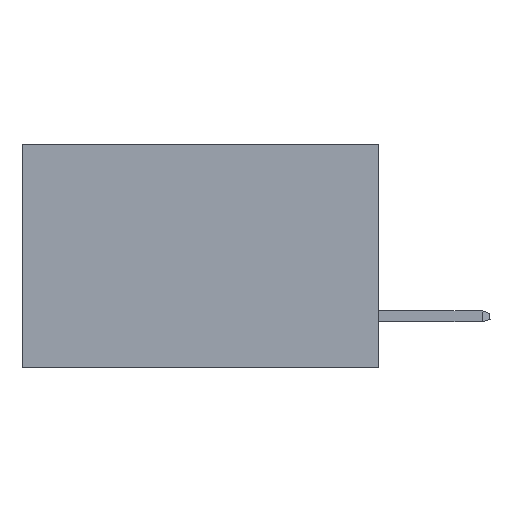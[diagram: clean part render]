
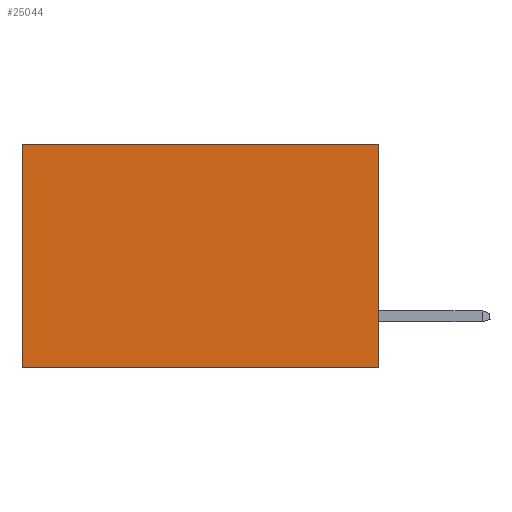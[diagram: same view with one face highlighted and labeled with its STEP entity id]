
A CAD part, left-side view. The second image highlights one B-rep face of the part: STEP entity #25044.
In plain terms, the highlighted planar face has unit normal (-1, 0, 0).
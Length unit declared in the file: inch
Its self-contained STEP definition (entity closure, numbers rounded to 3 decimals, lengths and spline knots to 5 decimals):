
#1061 = ORIENTED_EDGE ( 'NONE', *, *, #13146, .F. ) ;
#1868 = LINE ( 'NONE', #22021, #13992 ) ;
#2706 = CARTESIAN_POINT ( 'NONE',  ( 0.277, 0., 0. ) ) ;
#2955 = DIRECTION ( 'NONE',  ( 1., 0., 0. ) ) ;
#3081 = VERTEX_POINT ( 'NONE', #17607 ) ;
#4212 = VECTOR ( 'NONE', #24711, 39.37008 ) ;
#4604 = LINE ( 'NONE', #2706, #22909 ) ;
#5307 = EDGE_CURVE ( 'NONE', #3081, #27605, #1868, .T. ) ;
#7380 = CARTESIAN_POINT ( 'NONE',  ( 0.277, 0., 0. ) ) ;
#9707 = ORIENTED_EDGE ( 'NONE', *, *, #5307, .T. ) ;
#9942 = EDGE_CURVE ( 'NONE', #21710, #3081, #4604, .T. ) ;
#10630 = VECTOR ( 'NONE', #27394, 39.37008 ) ;
#10863 = FACE_OUTER_BOUND ( 'NONE', #11368, .T. ) ;
#10895 = CARTESIAN_POINT ( 'NONE',  ( 0.277, 0., -0.37 ) ) ;
#11368 = EDGE_LOOP ( 'NONE', ( #9707, #1061, #27638, #25913 ) ) ;
#13146 = EDGE_CURVE ( 'NONE', #21441, #27605, #15527, .T. ) ;
#13992 = VECTOR ( 'NONE', #22267, 39.37008 ) ;
#15527 = LINE ( 'NONE', #10895, #10630 ) ;
#17388 = PLANE ( 'NONE',  #29393 ) ;
#17607 = CARTESIAN_POINT ( 'NONE',  ( 0.277, 0.59, 0. ) ) ;
#19135 = CARTESIAN_POINT ( 'NONE',  ( 0.277, 0.59, -0.37 ) ) ;
#19759 = DIRECTION ( 'NONE',  ( 0., 0., -1. ) ) ;
#20055 = EDGE_CURVE ( 'NONE', #21710, #21441, #23262, .T. ) ;
#21441 = VERTEX_POINT ( 'NONE', #29911 ) ;
#21710 = VERTEX_POINT ( 'NONE', #7380 ) ;
#21877 = DIRECTION ( 'NONE',  ( 0., 1., 0. ) ) ;
#22021 = CARTESIAN_POINT ( 'NONE',  ( 0.277, 0.59, -0.37 ) ) ;
#22267 = DIRECTION ( 'NONE',  ( 0., 0., -1. ) ) ;
#22347 = CARTESIAN_POINT ( 'NONE',  ( 0.277, 0., -0.37 ) ) ;
#22909 = VECTOR ( 'NONE', #21877, 39.37008 ) ;
#23262 = LINE ( 'NONE', #22347, #4212 ) ;
#24711 = DIRECTION ( 'NONE',  ( 0., 0., -1. ) ) ;
#25044 = ADVANCED_FACE ( 'NONE', ( #10863 ), #17388, .F. ) ;
#25913 = ORIENTED_EDGE ( 'NONE', *, *, #9942, .T. ) ;
#27394 = DIRECTION ( 'NONE',  ( 0., 1., 0. ) ) ;
#27605 = VERTEX_POINT ( 'NONE', #19135 ) ;
#27638 = ORIENTED_EDGE ( 'NONE', *, *, #20055, .F. ) ;
#28978 = CARTESIAN_POINT ( 'NONE',  ( 0.277, 0., -0.37 ) ) ;
#29393 = AXIS2_PLACEMENT_3D ( 'NONE', #28978, #2955, #19759 ) ;
#29911 = CARTESIAN_POINT ( 'NONE',  ( 0.277, 0., -0.37 ) ) ;
